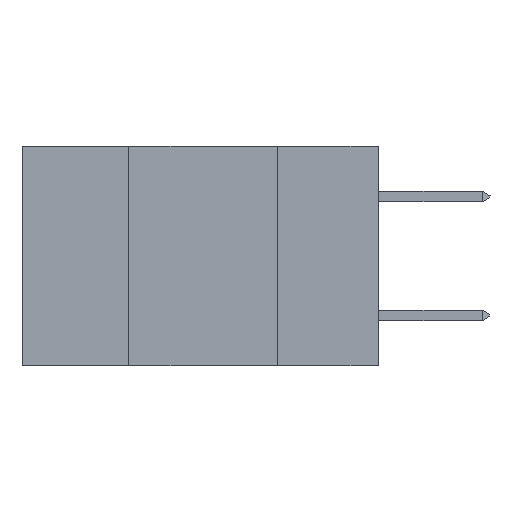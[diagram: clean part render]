
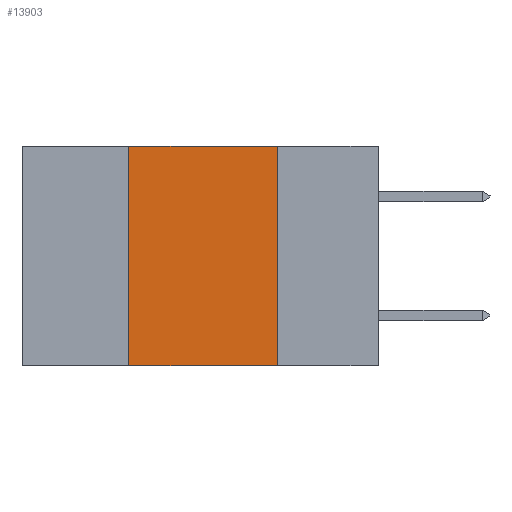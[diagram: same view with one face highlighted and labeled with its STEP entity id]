
A CAD part, left-side view. The second image highlights one B-rep face of the part: STEP entity #13903.
In plain terms, the highlighted planar face has unit normal (-1, 0, 0).
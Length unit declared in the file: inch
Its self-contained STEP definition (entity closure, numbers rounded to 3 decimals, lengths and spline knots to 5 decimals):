
#130 = VECTOR ( 'NONE', #6343, 39.37008 ) ;
#929 = LINE ( 'NONE', #16555, #12344 ) ;
#1071 = CARTESIAN_POINT ( 'NONE',  ( 0., 0.6, -0.37 ) ) ;
#1346 = CARTESIAN_POINT ( 'NONE',  ( 0., 0.17, 0. ) ) ;
#2293 = CARTESIAN_POINT ( 'NONE',  ( 0., 0.6, 0. ) ) ;
#2309 = DIRECTION ( 'NONE',  ( 0., 0., -1. ) ) ;
#2716 = EDGE_CURVE ( 'NONE', #13379, #7240, #9368, .T. ) ;
#3462 = EDGE_LOOP ( 'NONE', ( #5867, #13306, #4489, #9532 ) ) ;
#3964 = CARTESIAN_POINT ( 'NONE',  ( 0., 0.42, -0.37 ) ) ;
#4279 = PLANE ( 'NONE',  #4626 ) ;
#4489 = ORIENTED_EDGE ( 'NONE', *, *, #2716, .F. ) ;
#4626 = AXIS2_PLACEMENT_3D ( 'NONE', #10611, #5405, #11894 ) ;
#4702 = VERTEX_POINT ( 'NONE', #12517 ) ;
#5134 = LINE ( 'NONE', #2293, #130 ) ;
#5405 = DIRECTION ( 'NONE',  ( 1., 0., 0. ) ) ;
#5867 = ORIENTED_EDGE ( 'NONE', *, *, #6488, .F. ) ;
#6343 = DIRECTION ( 'NONE',  ( 0., -1., 0. ) ) ;
#6488 = EDGE_CURVE ( 'NONE', #14262, #4702, #929, .T. ) ;
#7240 = VERTEX_POINT ( 'NONE', #10750 ) ;
#7824 = VECTOR ( 'NONE', #13331, 39.37008 ) ;
#8350 = EDGE_CURVE ( 'NONE', #13379, #4702, #12982, .T. ) ;
#9368 = LINE ( 'NONE', #11873, #7824 ) ;
#9532 = ORIENTED_EDGE ( 'NONE', *, *, #8350, .T. ) ;
#10611 = CARTESIAN_POINT ( 'NONE',  ( 0., 0.6, 0. ) ) ;
#10750 = CARTESIAN_POINT ( 'NONE',  ( 0., 0.42, 0. ) ) ;
#10858 = FACE_OUTER_BOUND ( 'NONE', #3462, .T. ) ;
#11873 = CARTESIAN_POINT ( 'NONE',  ( 0., 0.42, -0.37 ) ) ;
#11894 = DIRECTION ( 'NONE',  ( 0., 0., -1. ) ) ;
#12344 = VECTOR ( 'NONE', #2309, 39.37008 ) ;
#12517 = CARTESIAN_POINT ( 'NONE',  ( 0., 0.17, -0.37 ) ) ;
#12982 = LINE ( 'NONE', #1071, #14531 ) ;
#13306 = ORIENTED_EDGE ( 'NONE', *, *, #14207, .F. ) ;
#13331 = DIRECTION ( 'NONE',  ( 0., 0., 1. ) ) ;
#13379 = VERTEX_POINT ( 'NONE', #3964 ) ;
#13903 = ADVANCED_FACE ( 'NONE', ( #10858 ), #4279, .F. ) ;
#14207 = EDGE_CURVE ( 'NONE', #7240, #14262, #5134, .T. ) ;
#14262 = VERTEX_POINT ( 'NONE', #1346 ) ;
#14531 = VECTOR ( 'NONE', #15400, 39.37008 ) ;
#15400 = DIRECTION ( 'NONE',  ( 0., -1., 0. ) ) ;
#16555 = CARTESIAN_POINT ( 'NONE',  ( 0., 0.17, -0.37 ) ) ;
